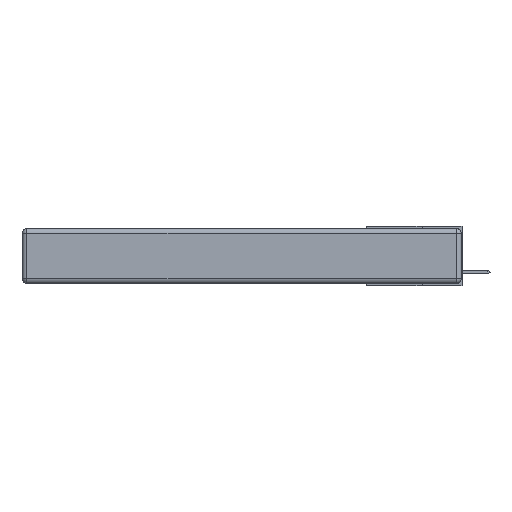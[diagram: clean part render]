
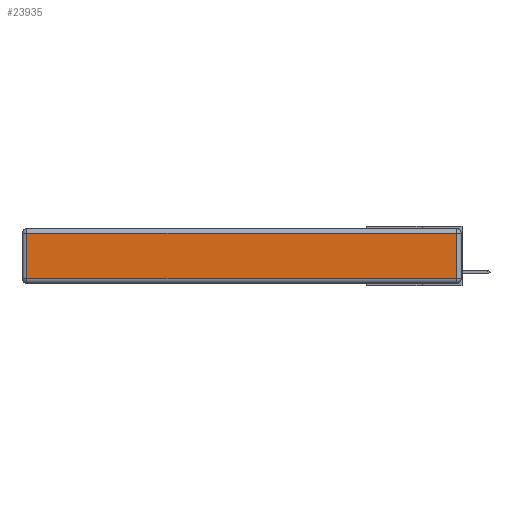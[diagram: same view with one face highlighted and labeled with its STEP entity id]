
A CAD part, left-side view. The second image highlights one B-rep face of the part: STEP entity #23935.
In plain terms, the highlighted planar face has unit normal (-1, 0, 0).
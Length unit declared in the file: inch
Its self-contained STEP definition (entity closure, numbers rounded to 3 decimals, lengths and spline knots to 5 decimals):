
#268 = EDGE_CURVE ( 'NONE', #23305, #4132, #24056, .T. ) ;
#1447 = EDGE_CURVE ( 'NONE', #20878, #4349, #10960, .T. ) ;
#1825 = DIRECTION ( 'NONE',  ( 0., 0., -1. ) ) ;
#1997 = VECTOR ( 'NONE', #1825, 39.37008 ) ;
#2048 = ORIENTED_EDGE ( 'NONE', *, *, #1447, .T. ) ;
#3364 = FACE_OUTER_BOUND ( 'NONE', #10996, .T. ) ;
#3728 = DIRECTION ( 'NONE',  ( -1., 0., 0. ) ) ;
#4132 = VERTEX_POINT ( 'NONE', #22209 ) ;
#4349 = VERTEX_POINT ( 'NONE', #19588 ) ;
#4867 = VECTOR ( 'NONE', #20025, 39.37008 ) ;
#6291 = ORIENTED_EDGE ( 'NONE', *, *, #19035, .T. ) ;
#9256 = LINE ( 'NONE', #20872, #1997 ) ;
#9777 = AXIS2_PLACEMENT_3D ( 'NONE', #24564, #3728, #20981 ) ;
#10277 = CARTESIAN_POINT ( 'NONE',  ( 0., 0.03, -0.343 ) ) ;
#10960 = LINE ( 'NONE', #12651, #11271 ) ;
#10996 = EDGE_LOOP ( 'NONE', ( #2048, #12474, #22476, #6291 ) ) ;
#11271 = VECTOR ( 'NONE', #14570, 39.37008 ) ;
#12474 = ORIENTED_EDGE ( 'NONE', *, *, #21977, .T. ) ;
#12651 = CARTESIAN_POINT ( 'NONE',  ( 0., 0., -0.313 ) ) ;
#13638 = CARTESIAN_POINT ( 'NONE',  ( 0., 2.72, -0.313 ) ) ;
#14570 = DIRECTION ( 'NONE',  ( 0., -1., 0. ) ) ;
#15197 = PLANE ( 'NONE',  #9777 ) ;
#16476 = DIRECTION ( 'NONE',  ( 0., 1., 0. ) ) ;
#19035 = EDGE_CURVE ( 'NONE', #4132, #20878, #9256, .T. ) ;
#19588 = CARTESIAN_POINT ( 'NONE',  ( 0., 0.03, -0.313 ) ) ;
#20025 = DIRECTION ( 'NONE',  ( 0., 0., 1. ) ) ;
#20474 = CARTESIAN_POINT ( 'NONE',  ( 0., 2.75, -0.03 ) ) ;
#20872 = CARTESIAN_POINT ( 'NONE',  ( 0., 2.72, -0.343 ) ) ;
#20878 = VERTEX_POINT ( 'NONE', #13638 ) ;
#20981 = DIRECTION ( 'NONE',  ( 0., 0., 1. ) ) ;
#21694 = LINE ( 'NONE', #10277, #4867 ) ;
#21745 = CARTESIAN_POINT ( 'NONE',  ( 0., 0.03, -0.03 ) ) ;
#21977 = EDGE_CURVE ( 'NONE', #4349, #23305, #21694, .T. ) ;
#22209 = CARTESIAN_POINT ( 'NONE',  ( 0., 2.72, -0.03 ) ) ;
#22476 = ORIENTED_EDGE ( 'NONE', *, *, #268, .T. ) ;
#23305 = VERTEX_POINT ( 'NONE', #21745 ) ;
#23439 = VECTOR ( 'NONE', #16476, 39.37008 ) ;
#23935 = ADVANCED_FACE ( 'NONE', ( #3364 ), #15197, .T. ) ;
#24056 = LINE ( 'NONE', #20474, #23439 ) ;
#24564 = CARTESIAN_POINT ( 'NONE',  ( 0., 0., -0.343 ) ) ;
